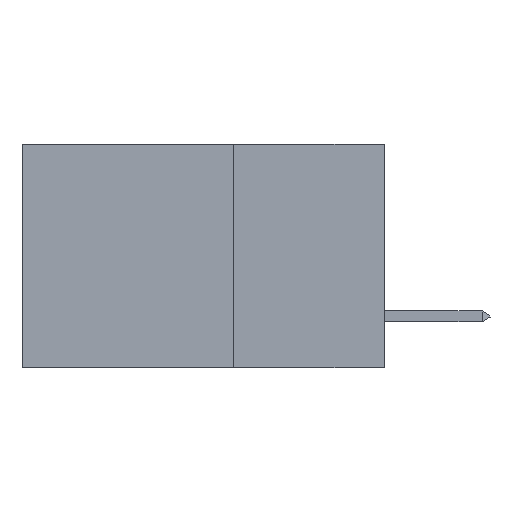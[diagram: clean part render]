
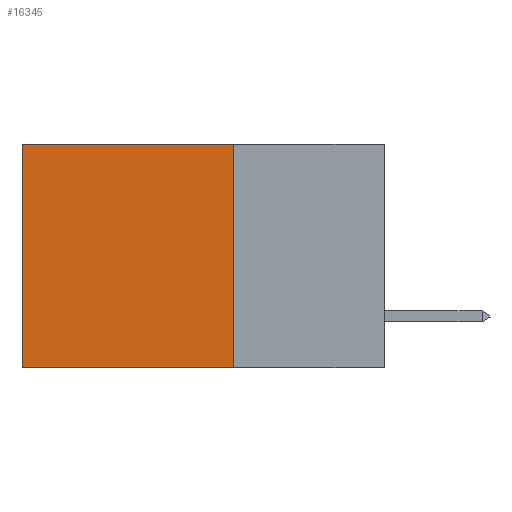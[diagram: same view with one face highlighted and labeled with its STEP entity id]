
A CAD part, left-side view. The second image highlights one B-rep face of the part: STEP entity #16345.
In plain terms, the highlighted planar face has unit normal (-1, 0, 0).
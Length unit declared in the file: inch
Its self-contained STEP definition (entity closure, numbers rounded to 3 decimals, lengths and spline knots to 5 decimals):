
#1568 = VECTOR ( 'NONE', #18881, 39.37008 ) ;
#2495 = CARTESIAN_POINT ( 'NONE',  ( 0.2875, 0.6, -0.37 ) ) ;
#3099 = DIRECTION ( 'NONE',  ( 0., 1., 0. ) ) ;
#3258 = FACE_OUTER_BOUND ( 'NONE', #22969, .T. ) ;
#3717 = DIRECTION ( 'NONE',  ( 1., 0., 0. ) ) ;
#3750 = ORIENTED_EDGE ( 'NONE', *, *, #22439, .T. ) ;
#4298 = DIRECTION ( 'NONE',  ( 0., 1., 0. ) ) ;
#4613 = LINE ( 'NONE', #20206, #27203 ) ;
#4926 = DIRECTION ( 'NONE',  ( 0., 0., -1. ) ) ;
#8976 = EDGE_CURVE ( 'NONE', #27958, #34079, #26614, .T. ) ;
#11220 = ORIENTED_EDGE ( 'NONE', *, *, #26255, .T. ) ;
#11290 = CARTESIAN_POINT ( 'NONE',  ( 0.2875, 0.25, -0.37 ) ) ;
#11535 = LINE ( 'NONE', #20762, #16893 ) ;
#13100 = CARTESIAN_POINT ( 'NONE',  ( 0.2875, 0.25, 0. ) ) ;
#15335 = LINE ( 'NONE', #13100, #1568 ) ;
#16345 = ADVANCED_FACE ( 'NONE', ( #3258 ), #29257, .F. ) ;
#16893 = VECTOR ( 'NONE', #4298, 39.37008 ) ;
#18881 = DIRECTION ( 'NONE',  ( 0., 0., -1. ) ) ;
#20165 = CARTESIAN_POINT ( 'NONE',  ( 0.2875, 0.25, -0.37 ) ) ;
#20206 = CARTESIAN_POINT ( 'NONE',  ( 0.2875, 0.6, 0. ) ) ;
#20762 = CARTESIAN_POINT ( 'NONE',  ( 0.2875, 0.25, 0. ) ) ;
#20784 = ORIENTED_EDGE ( 'NONE', *, *, #8976, .F. ) ;
#22439 = EDGE_CURVE ( 'NONE', #26413, #23209, #11535, .T. ) ;
#22969 = EDGE_LOOP ( 'NONE', ( #11220, #20784, #33569, #3750 ) ) ;
#23209 = VERTEX_POINT ( 'NONE', #35353 ) ;
#24444 = VECTOR ( 'NONE', #3099, 39.37008 ) ;
#25768 = EDGE_CURVE ( 'NONE', #26413, #27958, #15335, .T. ) ;
#26255 = EDGE_CURVE ( 'NONE', #23209, #34079, #4613, .T. ) ;
#26413 = VERTEX_POINT ( 'NONE', #26778 ) ;
#26614 = LINE ( 'NONE', #11290, #24444 ) ;
#26778 = CARTESIAN_POINT ( 'NONE',  ( 0.2875, 0.25, 0. ) ) ;
#27203 = VECTOR ( 'NONE', #4926, 39.37008 ) ;
#27958 = VERTEX_POINT ( 'NONE', #20165 ) ;
#29257 = PLANE ( 'NONE',  #31530 ) ;
#31530 = AXIS2_PLACEMENT_3D ( 'NONE', #35026, #3717, #32059 ) ;
#32059 = DIRECTION ( 'NONE',  ( 0., 0., -1. ) ) ;
#33569 = ORIENTED_EDGE ( 'NONE', *, *, #25768, .F. ) ;
#34079 = VERTEX_POINT ( 'NONE', #2495 ) ;
#35026 = CARTESIAN_POINT ( 'NONE',  ( 0.2875, 0.25, 0. ) ) ;
#35353 = CARTESIAN_POINT ( 'NONE',  ( 0.2875, 0.6, 0. ) ) ;
